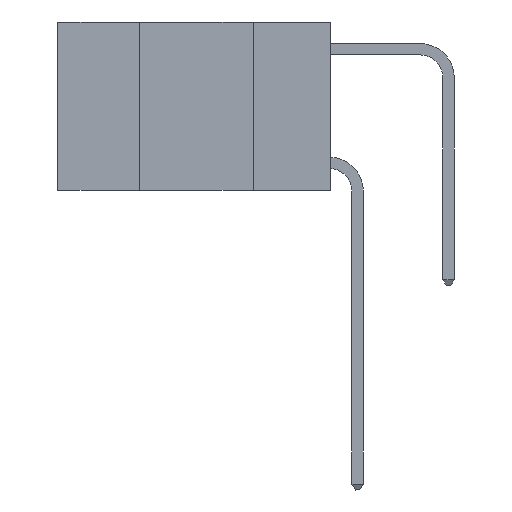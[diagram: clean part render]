
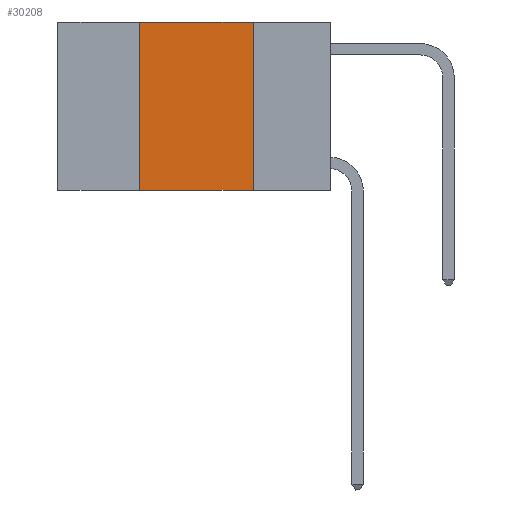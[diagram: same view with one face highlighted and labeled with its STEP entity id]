
A CAD part, left-side view. The second image highlights one B-rep face of the part: STEP entity #30208.
In plain terms, the highlighted planar face has unit normal (-1, 0, 0).
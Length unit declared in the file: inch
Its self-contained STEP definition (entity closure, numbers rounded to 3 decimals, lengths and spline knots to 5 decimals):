
#654 = ORIENTED_EDGE ( 'NONE', *, *, #23390, .F. ) ;
#1506 = VERTEX_POINT ( 'NONE', #30270 ) ;
#2525 = DIRECTION ( 'NONE',  ( 0., -1., 0. ) ) ;
#3558 = LINE ( 'NONE', #11412, #6823 ) ;
#4302 = VERTEX_POINT ( 'NONE', #31576 ) ;
#5503 = ORIENTED_EDGE ( 'NONE', *, *, #9534, .F. ) ;
#5774 = VECTOR ( 'NONE', #10745, 39.37008 ) ;
#6065 = DIRECTION ( 'NONE',  ( 0., 0., -1. ) ) ;
#6823 = VECTOR ( 'NONE', #31588, 39.37008 ) ;
#7116 = CARTESIAN_POINT ( 'NONE',  ( 0., 0.42, -0.37 ) ) ;
#7486 = EDGE_CURVE ( 'NONE', #25941, #1506, #3558, .T. ) ;
#7532 = CARTESIAN_POINT ( 'NONE',  ( 0., 0.42, 0. ) ) ;
#8160 = EDGE_LOOP ( 'NONE', ( #30756, #5503, #654, #30155 ) ) ;
#8844 = CARTESIAN_POINT ( 'NONE',  ( 0., 0.17, 0. ) ) ;
#9534 = EDGE_CURVE ( 'NONE', #15062, #4302, #15010, .T. ) ;
#9870 = DIRECTION ( 'NONE',  ( 0., 0., -1. ) ) ;
#10381 = CARTESIAN_POINT ( 'NONE',  ( 0., 0.6, 0. ) ) ;
#10745 = DIRECTION ( 'NONE',  ( 0., 0., 1. ) ) ;
#10963 = LINE ( 'NONE', #8844, #18786 ) ;
#11412 = CARTESIAN_POINT ( 'NONE',  ( 0., 0.6, -0.37 ) ) ;
#12604 = VECTOR ( 'NONE', #2525, 39.37008 ) ;
#15010 = LINE ( 'NONE', #10381, #12604 ) ;
#15062 = VERTEX_POINT ( 'NONE', #7532 ) ;
#15514 = LINE ( 'NONE', #25523, #5774 ) ;
#18786 = VECTOR ( 'NONE', #6065, 39.37008 ) ;
#20158 = AXIS2_PLACEMENT_3D ( 'NONE', #32355, #32024, #9870 ) ;
#20997 = EDGE_CURVE ( 'NONE', #4302, #1506, #10963, .T. ) ;
#22021 = FACE_OUTER_BOUND ( 'NONE', #8160, .T. ) ;
#23390 = EDGE_CURVE ( 'NONE', #25941, #15062, #15514, .T. ) ;
#25523 = CARTESIAN_POINT ( 'NONE',  ( 0., 0.42, 0. ) ) ;
#25941 = VERTEX_POINT ( 'NONE', #7116 ) ;
#29589 = PLANE ( 'NONE',  #20158 ) ;
#30155 = ORIENTED_EDGE ( 'NONE', *, *, #7486, .T. ) ;
#30208 = ADVANCED_FACE ( 'NONE', ( #22021 ), #29589, .F. ) ;
#30270 = CARTESIAN_POINT ( 'NONE',  ( 0., 0.17, -0.37 ) ) ;
#30756 = ORIENTED_EDGE ( 'NONE', *, *, #20997, .F. ) ;
#31576 = CARTESIAN_POINT ( 'NONE',  ( 0., 0.17, 0. ) ) ;
#31588 = DIRECTION ( 'NONE',  ( 0., -1., 0. ) ) ;
#32024 = DIRECTION ( 'NONE',  ( 1., 0., 0. ) ) ;
#32355 = CARTESIAN_POINT ( 'NONE',  ( 0., 0.6, 0. ) ) ;
